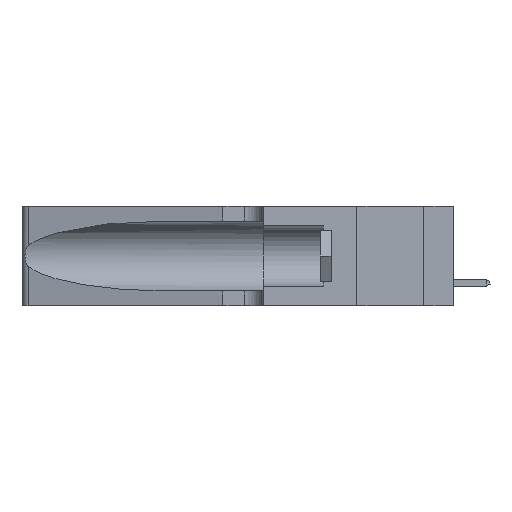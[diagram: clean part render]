
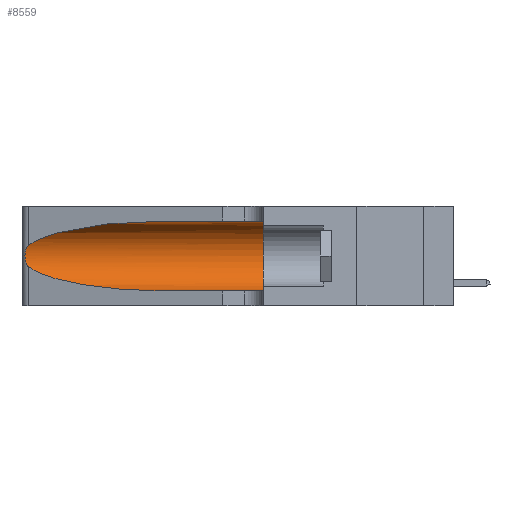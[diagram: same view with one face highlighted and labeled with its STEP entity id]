
A CAD part, left-side view. The second image highlights one B-rep face of the part: STEP entity #8559.
In plain terms, the highlighted cylindrical face has radius 3.308 mm (diameter 6.617 mm), a partial arc.
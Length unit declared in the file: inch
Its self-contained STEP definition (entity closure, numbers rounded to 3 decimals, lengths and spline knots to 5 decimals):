
#359 = ORIENTED_EDGE ( 'NONE', *, *, #16776, .F. ) ;
#536 = CARTESIAN_POINT ( 'NONE',  ( 0.25789, 1.23486, 0.15765 ) ) ;
#691 = CARTESIAN_POINT ( 'NONE',  ( 0.26018, 1.23835, 0.19895 ) ) ;
#732 = DIRECTION ( 'NONE',  ( 0., 0., 1. ) ) ;
#767 = CARTESIAN_POINT ( 'NONE',  ( 0.26017, 1.23833, 0.17102 ) ) ;
#805 = EDGE_CURVE ( 'NONE', #12266, #21819, #1821, .T. ) ;
#1540 = VECTOR ( 'NONE', #8281, 39.37008 ) ;
#1649 = CARTESIAN_POINT ( 'NONE',  ( 0.18966, 0.96281, 0.05475 ) ) ;
#1821 = LINE ( 'NONE', #6464, #1540 ) ;
#2259 = CARTESIAN_POINT ( 'NONE',  ( 0.26075, 1.23896, 0.178 ) ) ;
#2486 = CARTESIAN_POINT ( 'NONE',  ( 0.25487, 1.22718, 0.22369 ) ) ;
#3837 = CARTESIAN_POINT ( 'NONE',  ( 0.1305, 1.61858, 0.185 ) ) ;
#3998 =( BOUNDED_CURVE ( )  B_SPLINE_CURVE ( 3, ( #16092, #7083, #15851, #4990 ),
 .UNSPECIFIED., .F., .T. ) 
 B_SPLINE_CURVE_WITH_KNOTS ( ( 4, 4 ),
 ( 1.5708, 2.84003 ),
 .UNSPECIFIED. ) 
 CURVE ( )  GEOMETRIC_REPRESENTATION_ITEM ( )  RATIONAL_B_SPLINE_CURVE ( ( 1., 0.87, 0.87, 1. ) ) 
 REPRESENTATION_ITEM ( '' )  );
#4316 = CARTESIAN_POINT ( 'NONE',  ( 0.25787, 1.23484, 0.2124 ) ) ;
#4551 = ORIENTED_EDGE ( 'NONE', *, *, #20851, .T. ) ;
#4990 = CARTESIAN_POINT ( 'NONE',  ( 0.25487, 1.22718, 0.22369 ) ) ;
#5420 = ORIENTED_EDGE ( 'NONE', *, *, #7778, .T. ) ;
#5452 = VERTEX_POINT ( 'NONE', #11276 ) ;
#5974 = CARTESIAN_POINT ( 'NONE',  ( 0.1305, 0.35, 0.185 ) ) ;
#6067 = VERTEX_POINT ( 'NONE', #16451 ) ;
#6084 = FACE_OUTER_BOUND ( 'NONE', #14839, .T. ) ;
#6089 = CARTESIAN_POINT ( 'NONE',  ( 0.25854, 1.2359, 0.20912 ) ) ;
#6464 = CARTESIAN_POINT ( 'NONE',  ( 0.1305, 1.61858, 0.05475 ) ) ;
#6803 = CARTESIAN_POINT ( 'NONE',  ( 0.1305, 0.35, 0.05475 ) ) ;
#7003 = CARTESIAN_POINT ( 'NONE',  ( 0.1305, 0.72297, 0.05475 ) ) ;
#7083 = CARTESIAN_POINT ( 'NONE',  ( 0.18966, 0.96281, 0.31525 ) ) ;
#7523 = DIRECTION ( 'NONE',  ( 0., 0., -1. ) ) ;
#7778 = EDGE_CURVE ( 'NONE', #5452, #6067, #20832, .T. ) ;
#8209 = CIRCLE ( 'NONE', #22113, 0.13025 ) ;
#8281 = DIRECTION ( 'NONE',  ( 0., -1., 0. ) ) ;
#8285 = EDGE_CURVE ( 'NONE', #18072, #5452, #3998, .T. ) ;
#8559 = ADVANCED_FACE ( 'NONE', ( #6084 ), #10899, .F. ) ;
#8561 = ORIENTED_EDGE ( 'NONE', *, *, #8285, .T. ) ;
#9345 = DIRECTION ( 'NONE',  ( 0., -1., 0. ) ) ;
#9573 = VECTOR ( 'NONE', #22441, 39.37008 ) ;
#9659 = CARTESIAN_POINT ( 'NONE',  ( 0.25555, 1.22994, 0.2215 ) ) ;
#10779 = CARTESIAN_POINT ( 'NONE',  ( 0.25487, 1.22718, 0.14631 ) ) ;
#10899 = CYLINDRICAL_SURFACE ( 'NONE', #14287, 0.13025 ) ;
#11276 = CARTESIAN_POINT ( 'NONE',  ( 0.25487, 1.22718, 0.22369 ) ) ;
#11320 = CARTESIAN_POINT ( 'NONE',  ( 0.25555, 1.22993, 0.14849 ) ) ;
#11685 = ORIENTED_EDGE ( 'NONE', *, *, #14868, .F. ) ;
#12266 = VERTEX_POINT ( 'NONE', #7003 ) ;
#13116 = CARTESIAN_POINT ( 'NONE',  ( 0.25639, 1.23184, 0.21858 ) ) ;
#13277 = CARTESIAN_POINT ( 'NONE',  ( 0.25856, 1.23593, 0.16098 ) ) ;
#13348 = CARTESIAN_POINT ( 'NONE',  ( 0.25639, 1.23186, 0.15144 ) ) ;
#13465 = DIRECTION ( 'NONE',  ( 0., 1., 0. ) ) ;
#13524 = CARTESIAN_POINT ( 'NONE',  ( 0.1305, 1.61858, 0.31525 ) ) ;
#14287 = AXIS2_PLACEMENT_3D ( 'NONE', #3837, #9345, #7523 ) ;
#14839 = EDGE_LOOP ( 'NONE', ( #8561, #5420, #4551, #16860, #359, #11685 ) ) ;
#14868 = EDGE_CURVE ( 'NONE', #18072, #20830, #22820, .T. ) ;
#15250 = CARTESIAN_POINT ( 'NONE',  ( 0.25487, 1.22718, 0.14631 ) ) ;
#15851 = CARTESIAN_POINT ( 'NONE',  ( 0.2373, 1.15595, 0.28018 ) ) ;
#16092 = CARTESIAN_POINT ( 'NONE',  ( 0.1305, 0.72297, 0.31525 ) ) ;
#16451 = CARTESIAN_POINT ( 'NONE',  ( 0.25487, 1.22718, 0.14631 ) ) ;
#16776 = EDGE_CURVE ( 'NONE', #20830, #21819, #8209, .T. ) ;
#16860 = ORIENTED_EDGE ( 'NONE', *, *, #805, .T. ) ;
#18072 = VERTEX_POINT ( 'NONE', #20940 ) ;
#19387 =( BOUNDED_CURVE ( )  B_SPLINE_CURVE ( 3, ( #10779, #19626, #1649, #21280 ),
 .UNSPECIFIED., .F., .F. ) 
 B_SPLINE_CURVE_WITH_KNOTS ( ( 4, 4 ),
 ( 3.44316, 4.71239 ),
 .UNSPECIFIED. ) 
 CURVE ( )  GEOMETRIC_REPRESENTATION_ITEM ( )  RATIONAL_B_SPLINE_CURVE ( ( 1., 0.87, 0.87, 1. ) ) 
 REPRESENTATION_ITEM ( '' )  );
#19626 = CARTESIAN_POINT ( 'NONE',  ( 0.2373, 1.15595, 0.08982 ) ) ;
#20634 = CARTESIAN_POINT ( 'NONE',  ( 0.26075, 1.23896, 0.19203 ) ) ;
#20830 = VERTEX_POINT ( 'NONE', #21510 ) ;
#20832 = B_SPLINE_CURVE_WITH_KNOTS ( 'NONE', 3,
 ( #2486, #9659, #13116, #4316, #6089, #691, #20634, #2259, #767, #13277, #536, #13348, #11320, #15250 ),
 .UNSPECIFIED., .F., .F.,
 ( 4, 2, 2, 2, 2, 2, 4 ),
 ( 0., 0.00027, 0.00053, 0.00107, 0.0016, 0.00187, 0.00214 ),
 .UNSPECIFIED. ) ;
#20851 = EDGE_CURVE ( 'NONE', #6067, #12266, #19387, .T. ) ;
#20940 = CARTESIAN_POINT ( 'NONE',  ( 0.1305, 0.72297, 0.31525 ) ) ;
#21280 = CARTESIAN_POINT ( 'NONE',  ( 0.1305, 0.72297, 0.05475 ) ) ;
#21510 = CARTESIAN_POINT ( 'NONE',  ( 0.1305, 0.35, 0.31525 ) ) ;
#21819 = VERTEX_POINT ( 'NONE', #6803 ) ;
#22113 = AXIS2_PLACEMENT_3D ( 'NONE', #5974, #13465, #732 ) ;
#22441 = DIRECTION ( 'NONE',  ( 0., -1., 0. ) ) ;
#22820 = LINE ( 'NONE', #13524, #9573 ) ;
